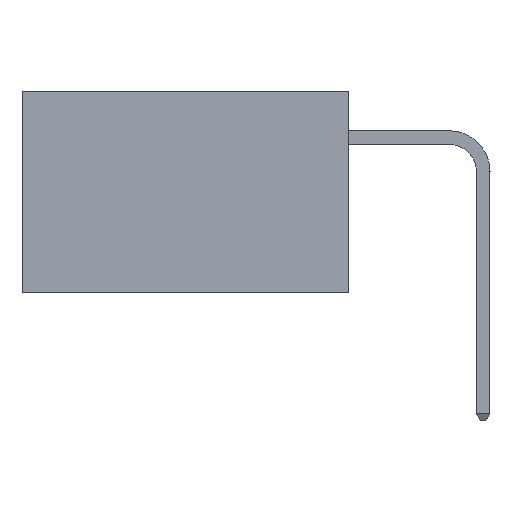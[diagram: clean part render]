
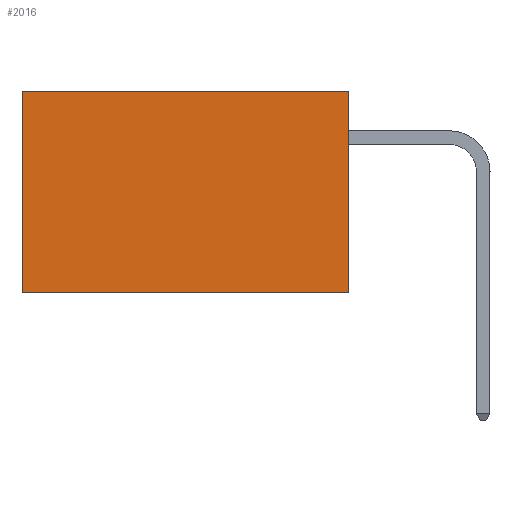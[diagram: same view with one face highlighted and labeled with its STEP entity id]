
A CAD part, left-side view. The second image highlights one B-rep face of the part: STEP entity #2016.
In plain terms, the highlighted planar face has unit normal (-1, 0, 0).
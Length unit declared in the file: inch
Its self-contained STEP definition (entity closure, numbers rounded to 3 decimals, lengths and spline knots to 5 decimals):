
#568 = DIRECTION ( 'NONE',  ( 0., 0., -1. ) ) ;
#787 = VECTOR ( 'NONE', #568, 39.37008 ) ;
#1318 = ORIENTED_EDGE ( 'NONE', *, *, #11933, .F. ) ;
#2009 = VECTOR ( 'NONE', #9628, 39.37008 ) ;
#2016 = ADVANCED_FACE ( 'NONE', ( #19407 ), #19954, .F. ) ;
#2080 = LINE ( 'NONE', #2205, #15178 ) ;
#2205 = CARTESIAN_POINT ( 'NONE',  ( 0.2875, 0., 0. ) ) ;
#3928 = ORIENTED_EDGE ( 'NONE', *, *, #10161, .F. ) ;
#5972 = ORIENTED_EDGE ( 'NONE', *, *, #19448, .T. ) ;
#7788 = DIRECTION ( 'NONE',  ( 1., 0., 0. ) ) ;
#7813 = CARTESIAN_POINT ( 'NONE',  ( 0.2875, 0., 0. ) ) ;
#8335 = EDGE_CURVE ( 'NONE', #15110, #11853, #15566, .T. ) ;
#9298 = DIRECTION ( 'NONE',  ( 0., 1., 0. ) ) ;
#9628 = DIRECTION ( 'NONE',  ( 0., 1., 0. ) ) ;
#10161 = EDGE_CURVE ( 'NONE', #17995, #11853, #20037, .T. ) ;
#11853 = VERTEX_POINT ( 'NONE', #16156 ) ;
#11933 = EDGE_CURVE ( 'NONE', #17133, #17995, #2080, .T. ) ;
#14543 = CARTESIAN_POINT ( 'NONE',  ( 0.2875, 0., -0.37 ) ) ;
#14956 = VECTOR ( 'NONE', #9298, 39.37008 ) ;
#14965 = ORIENTED_EDGE ( 'NONE', *, *, #8335, .T. ) ;
#15110 = VERTEX_POINT ( 'NONE', #21594 ) ;
#15178 = VECTOR ( 'NONE', #16359, 39.37008 ) ;
#15566 = LINE ( 'NONE', #18360, #787 ) ;
#16156 = CARTESIAN_POINT ( 'NONE',  ( 0.2875, 0.6, -0.37 ) ) ;
#16162 = LINE ( 'NONE', #7813, #2009 ) ;
#16359 = DIRECTION ( 'NONE',  ( 0., 0., -1. ) ) ;
#16444 = CARTESIAN_POINT ( 'NONE',  ( 0.2875, 0., 0. ) ) ;
#17133 = VERTEX_POINT ( 'NONE', #18955 ) ;
#17995 = VERTEX_POINT ( 'NONE', #19514 ) ;
#18261 = AXIS2_PLACEMENT_3D ( 'NONE', #16444, #7788, #22778 ) ;
#18360 = CARTESIAN_POINT ( 'NONE',  ( 0.2875, 0.6, 0. ) ) ;
#18955 = CARTESIAN_POINT ( 'NONE',  ( 0.2875, 0., 0. ) ) ;
#19181 = EDGE_LOOP ( 'NONE', ( #14965, #3928, #1318, #5972 ) ) ;
#19407 = FACE_OUTER_BOUND ( 'NONE', #19181, .T. ) ;
#19448 = EDGE_CURVE ( 'NONE', #17133, #15110, #16162, .T. ) ;
#19514 = CARTESIAN_POINT ( 'NONE',  ( 0.2875, 0., -0.37 ) ) ;
#19954 = PLANE ( 'NONE',  #18261 ) ;
#20037 = LINE ( 'NONE', #14543, #14956 ) ;
#21594 = CARTESIAN_POINT ( 'NONE',  ( 0.2875, 0.6, 0. ) ) ;
#22778 = DIRECTION ( 'NONE',  ( 0., 0., -1. ) ) ;
